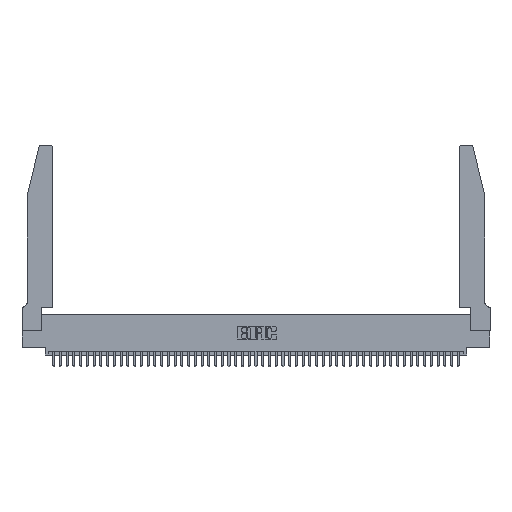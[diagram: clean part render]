
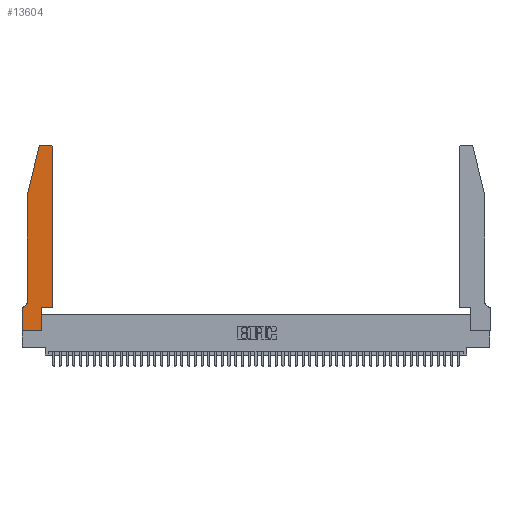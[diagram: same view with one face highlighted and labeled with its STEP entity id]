
A CAD part, top view. The second image highlights one B-rep face of the part: STEP entity #13604.
In plain terms, the highlighted planar face has unit normal (0, 0, 1).
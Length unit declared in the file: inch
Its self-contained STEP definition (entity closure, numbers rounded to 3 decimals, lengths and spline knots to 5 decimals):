
#872 = CIRCLE ( 'NONE', #23449, 0.03 ) ;
#1152 = ORIENTED_EDGE ( 'NONE', *, *, #32103, .T. ) ;
#1379 = FACE_OUTER_BOUND ( 'NONE', #5555, .T. ) ;
#1789 = CARTESIAN_POINT ( 'NONE',  ( 0.0755, 2., 0.37 ) ) ;
#2230 = CARTESIAN_POINT ( 'NONE',  ( 0.284, 2.72, 0.37 ) ) ;
#3758 = ORIENTED_EDGE ( 'NONE', *, *, #30763, .T. ) ;
#4116 = VERTEX_POINT ( 'NONE', #9160 ) ;
#4810 = LINE ( 'NONE', #28891, #13981 ) ;
#5453 = CARTESIAN_POINT ( 'NONE',  ( 0., 0., 0.37 ) ) ;
#5555 = EDGE_LOOP ( 'NONE', ( #43632, #10994, #3758, #33389, #42643, #22124, #30870, #1152, #22542, #41221, #8003, #32852 ) ) ;
#5837 = CARTESIAN_POINT ( 'NONE',  ( 0., 0., 0.37 ) ) ;
#6141 = DIRECTION ( 'NONE',  ( 1., 0., 0. ) ) ;
#6374 = EDGE_CURVE ( 'NONE', #26145, #24853, #13391, .T. ) ;
#7447 = CARTESIAN_POINT ( 'NONE',  ( 0.4505, 2.72, 0.37 ) ) ;
#7796 = DIRECTION ( 'NONE',  ( 0., -1., 0. ) ) ;
#7828 = VERTEX_POINT ( 'NONE', #5453 ) ;
#8003 = ORIENTED_EDGE ( 'NONE', *, *, #23445, .T. ) ;
#8479 = DIRECTION ( 'NONE',  ( 0., 0., 1. ) ) ;
#9073 = EDGE_CURVE ( 'NONE', #24909, #4116, #9652, .T. ) ;
#9160 = CARTESIAN_POINT ( 'NONE',  ( 0., 0.35, 0.37 ) ) ;
#9652 = LINE ( 'NONE', #33311, #38184 ) ;
#10994 = ORIENTED_EDGE ( 'NONE', *, *, #48862, .T. ) ;
#11355 = CARTESIAN_POINT ( 'NONE',  ( 0.2605, 2.75, 0.37 ) ) ;
#11529 = EDGE_CURVE ( 'NONE', #24853, #36102, #21627, .T. ) ;
#11572 = LINE ( 'NONE', #17227, #14039 ) ;
#11573 = CARTESIAN_POINT ( 'NONE',  ( 0.0755, 2., 0.37 ) ) ;
#12219 = PLANE ( 'NONE',  #36814 ) ;
#13391 = CIRCLE ( 'NONE', #28756, 0.03 ) ;
#13604 = ADVANCED_FACE ( 'NONE', ( #1379 ), #12219, .T. ) ;
#13710 = LINE ( 'NONE', #44412, #33147 ) ;
#13843 = CARTESIAN_POINT ( 'NONE',  ( 0.0755, 0.42, 0.37 ) ) ;
#13981 = VECTOR ( 'NONE', #32772, 39.37008 ) ;
#14039 = VECTOR ( 'NONE', #44300, 39.37008 ) ;
#15304 = VERTEX_POINT ( 'NONE', #1789 ) ;
#16150 = DIRECTION ( 'NONE',  ( 1., 0., 0. ) ) ;
#16838 = CIRCLE ( 'NONE', #46160, 0.07 ) ;
#17071 = CARTESIAN_POINT ( 'NONE',  ( 0.0055, 0.42, 0.37 ) ) ;
#17227 = CARTESIAN_POINT ( 'NONE',  ( 0.2865, 0.35, 0.37 ) ) ;
#17349 = VECTOR ( 'NONE', #41533, 39.37008 ) ;
#17395 = VECTOR ( 'NONE', #7796, 39.37008 ) ;
#18722 = VERTEX_POINT ( 'NONE', #45941 ) ;
#20291 = CARTESIAN_POINT ( 'NONE',  ( 0.2865, 0.35, 0.37 ) ) ;
#20410 = VECTOR ( 'NONE', #46123, 39.37008 ) ;
#21008 = DIRECTION ( 'NONE',  ( -1., 0., 0. ) ) ;
#21402 = DIRECTION ( 'NONE',  ( 0., -1., 0. ) ) ;
#21627 = LINE ( 'NONE', #11355, #20410 ) ;
#21731 = CARTESIAN_POINT ( 'NONE',  ( 0.0755, 2., 0.37 ) ) ;
#22124 = ORIENTED_EDGE ( 'NONE', *, *, #9073, .T. ) ;
#22127 = EDGE_CURVE ( 'NONE', #4116, #7828, #41123, .T. ) ;
#22542 = ORIENTED_EDGE ( 'NONE', *, *, #44962, .T. ) ;
#22698 = EDGE_CURVE ( 'NONE', #48860, #24909, #16838, .T. ) ;
#23445 = EDGE_CURVE ( 'NONE', #38576, #26145, #13710, .T. ) ;
#23449 = AXIS2_PLACEMENT_3D ( 'NONE', #2230, #29488, #6141 ) ;
#24853 = VERTEX_POINT ( 'NONE', #30731 ) ;
#24909 = VERTEX_POINT ( 'NONE', #39310 ) ;
#26145 = VERTEX_POINT ( 'NONE', #7447 ) ;
#27521 = VECTOR ( 'NONE', #37099, 39.37008 ) ;
#28752 = LINE ( 'NONE', #21731, #27521 ) ;
#28756 = AXIS2_PLACEMENT_3D ( 'NONE', #31790, #8479, #35672 ) ;
#28891 = CARTESIAN_POINT ( 'NONE',  ( 0.4505, 0.35, 0.37 ) ) ;
#28938 = EDGE_CURVE ( 'NONE', #15304, #48860, #49526, .T. ) ;
#29132 = VERTEX_POINT ( 'NONE', #20291 ) ;
#29488 = DIRECTION ( 'NONE',  ( 0., 0., 1. ) ) ;
#30731 = CARTESIAN_POINT ( 'NONE',  ( 0.4205, 2.75, 0.37 ) ) ;
#30763 = EDGE_CURVE ( 'NONE', #18722, #15304, #28752, .T. ) ;
#30861 = VECTOR ( 'NONE', #21402, 39.37008 ) ;
#30870 = ORIENTED_EDGE ( 'NONE', *, *, #22127, .T. ) ;
#31790 = CARTESIAN_POINT ( 'NONE',  ( 0.4205, 2.72, 0.37 ) ) ;
#32103 = EDGE_CURVE ( 'NONE', #7828, #40486, #37935, .T. ) ;
#32772 = DIRECTION ( 'NONE',  ( 1., 0., 0. ) ) ;
#32852 = ORIENTED_EDGE ( 'NONE', *, *, #6374, .T. ) ;
#33147 = VECTOR ( 'NONE', #48348, 39.37008 ) ;
#33311 = CARTESIAN_POINT ( 'NONE',  ( 0.0755, 0.35, 0.37 ) ) ;
#33389 = ORIENTED_EDGE ( 'NONE', *, *, #28938, .T. ) ;
#33958 = CARTESIAN_POINT ( 'NONE',  ( 0., 0., 0.37 ) ) ;
#34683 = CARTESIAN_POINT ( 'NONE',  ( 0.4505, 0.35, 0.37 ) ) ;
#34747 = EDGE_CURVE ( 'NONE', #29132, #38576, #4810, .T. ) ;
#35305 = CARTESIAN_POINT ( 'NONE',  ( 0., 0.35, 0.37 ) ) ;
#35672 = DIRECTION ( 'NONE',  ( 1., 0., 0. ) ) ;
#36102 = VERTEX_POINT ( 'NONE', #42321 ) ;
#36814 = AXIS2_PLACEMENT_3D ( 'NONE', #35305, #39337, #16150 ) ;
#37099 = DIRECTION ( 'NONE',  ( -0.239, -0.971, 0. ) ) ;
#37935 = LINE ( 'NONE', #33958, #17349 ) ;
#38184 = VECTOR ( 'NONE', #40887, 39.37008 ) ;
#38576 = VERTEX_POINT ( 'NONE', #34683 ) ;
#39310 = CARTESIAN_POINT ( 'NONE',  ( 0.0055, 0.35, 0.37 ) ) ;
#39337 = DIRECTION ( 'NONE',  ( 0., 0., 1. ) ) ;
#40486 = VERTEX_POINT ( 'NONE', #49948 ) ;
#40887 = DIRECTION ( 'NONE',  ( -1., 0., 0. ) ) ;
#41123 = LINE ( 'NONE', #5837, #30861 ) ;
#41221 = ORIENTED_EDGE ( 'NONE', *, *, #34747, .T. ) ;
#41533 = DIRECTION ( 'NONE',  ( 1., 0., 0. ) ) ;
#42321 = CARTESIAN_POINT ( 'NONE',  ( 0.284, 2.75, 0.37 ) ) ;
#42643 = ORIENTED_EDGE ( 'NONE', *, *, #22698, .T. ) ;
#43632 = ORIENTED_EDGE ( 'NONE', *, *, #11529, .T. ) ;
#44134 = DIRECTION ( 'NONE',  ( 0., 0., -1. ) ) ;
#44300 = DIRECTION ( 'NONE',  ( 0., 1., 0. ) ) ;
#44412 = CARTESIAN_POINT ( 'NONE',  ( 0.4505, 0.35, 0.37 ) ) ;
#44962 = EDGE_CURVE ( 'NONE', #40486, #29132, #11572, .T. ) ;
#45941 = CARTESIAN_POINT ( 'NONE',  ( 0.25487, 2.72718, 0.37 ) ) ;
#46123 = DIRECTION ( 'NONE',  ( -1., 0., 0. ) ) ;
#46160 = AXIS2_PLACEMENT_3D ( 'NONE', #17071, #44134, #21008 ) ;
#48348 = DIRECTION ( 'NONE',  ( 0., 1., 0. ) ) ;
#48860 = VERTEX_POINT ( 'NONE', #13843 ) ;
#48862 = EDGE_CURVE ( 'NONE', #36102, #18722, #872, .T. ) ;
#49526 = LINE ( 'NONE', #11573, #17395 ) ;
#49948 = CARTESIAN_POINT ( 'NONE',  ( 0.2865, 0., 0.37 ) ) ;
